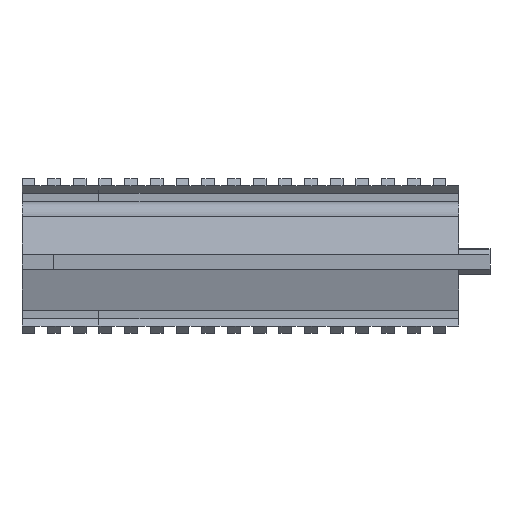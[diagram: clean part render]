
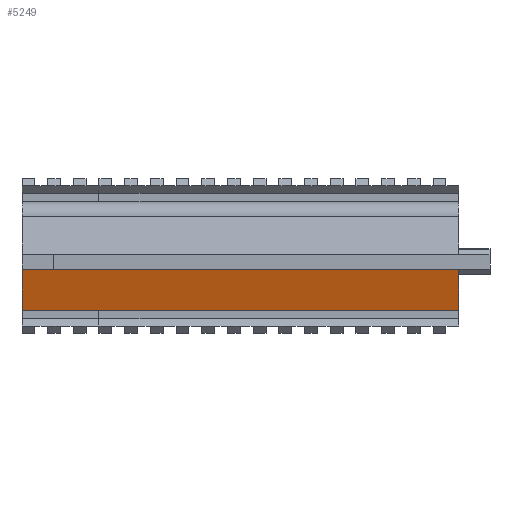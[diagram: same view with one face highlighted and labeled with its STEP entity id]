
A CAD part, left-side view. The second image highlights one B-rep face of the part: STEP entity #5249.
In plain terms, the highlighted planar face has unit normal (-0.956, 0, -0.294).
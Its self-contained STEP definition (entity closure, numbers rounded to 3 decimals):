
#314=FACE_OUTER_BOUND('',#593,.T.);
#593=EDGE_LOOP('',(#4600,#4601,#4602,#4603,#4604));
#1215=LINE('',#8116,#1930);
#1236=LINE('',#8165,#1951);
#1272=LINE('',#8246,#1987);
#1290=LINE('',#8294,#2005);
#1291=LINE('',#8295,#2006);
#1930=VECTOR('',#6648,10.);
#1951=VECTOR('',#6691,10.);
#1987=VECTOR('',#6759,10.);
#2005=VECTOR('',#6807,10.);
#2006=VECTOR('',#6808,10.);
#2425=VERTEX_POINT('',#8113);
#2426=VERTEX_POINT('',#8115);
#2443=VERTEX_POINT('',#8163);
#2472=VERTEX_POINT('',#8244);
#2487=VERTEX_POINT('',#8293);
#3114=EDGE_CURVE('',#2426,#2425,#1215,.T.);
#3139=EDGE_CURVE('',#2425,#2443,#1236,.T.);
#3179=EDGE_CURVE('',#2472,#2443,#1272,.T.);
#3203=EDGE_CURVE('',#2426,#2487,#1290,.T.);
#3204=EDGE_CURVE('',#2487,#2472,#1291,.T.);
#4600=ORIENTED_EDGE('',*,*,#3203,.F.);
#4601=ORIENTED_EDGE('',*,*,#3114,.T.);
#4602=ORIENTED_EDGE('',*,*,#3139,.T.);
#4603=ORIENTED_EDGE('',*,*,#3179,.F.);
#4604=ORIENTED_EDGE('',*,*,#3204,.F.);
#4975=PLANE('',#5559);
#5249=ADVANCED_FACE('',(#314),#4975,.T.);
#5559=AXIS2_PLACEMENT_3D('',#8292,#6805,#6806);
#6648=DIRECTION('',(0.,1.,0.));
#6691=DIRECTION('',(0.,1.,0.));
#6759=DIRECTION('',(-0.294,0.,0.956));
#6805=DIRECTION('center_axis',(-0.956,0.,-0.294));
#6806=DIRECTION('ref_axis',(-0.294,0.,0.956));
#6807=DIRECTION('',(0.294,0.,-0.956));
#6808=DIRECTION('',(0.,1.,0.));
#8113=CARTESIAN_POINT('',(-17.78,336.14,3.81));
#8115=CARTESIAN_POINT('',(-17.78,171.04,3.81));
#8116=CARTESIAN_POINT('',(-17.78,158.34,3.81));
#8163=CARTESIAN_POINT('',(-17.78,348.84,3.81));
#8165=CARTESIAN_POINT('',(-17.78,158.34,3.81));
#8244=CARTESIAN_POINT('',(-12.7,348.84,-12.7));
#8246=CARTESIAN_POINT('',(-14.828,348.84,-5.784));
#8292=CARTESIAN_POINT('Origin',(-12.7,171.04,-12.7));
#8293=CARTESIAN_POINT('',(-12.7,171.04,-12.7));
#8294=CARTESIAN_POINT('',(-14.828,171.04,-5.784));
#8295=CARTESIAN_POINT('',(-12.7,171.04,-12.7));
